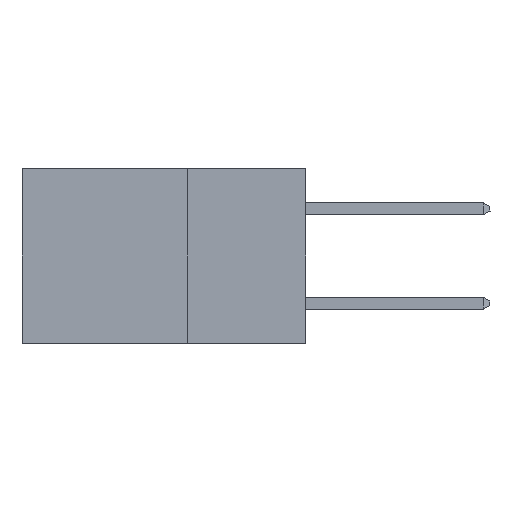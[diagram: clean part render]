
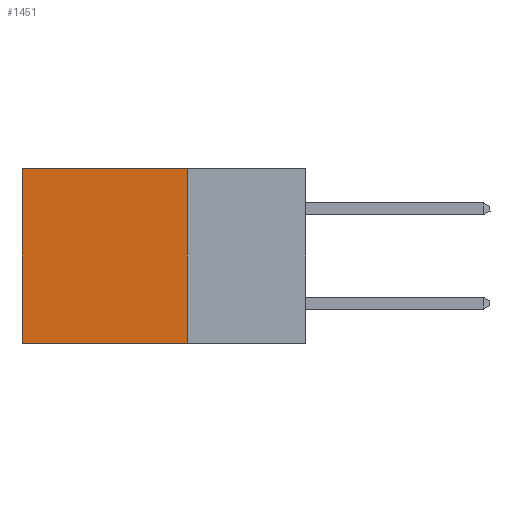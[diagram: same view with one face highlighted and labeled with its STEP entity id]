
A CAD part, left-side view. The second image highlights one B-rep face of the part: STEP entity #1451.
In plain terms, the highlighted planar face has unit normal (-1, 0, 0).
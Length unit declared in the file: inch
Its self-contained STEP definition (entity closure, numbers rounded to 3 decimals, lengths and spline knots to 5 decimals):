
#1451 = ADVANCED_FACE ( 'NONE', ( #2980 ), #4570, .F. ) ;
#2980 = FACE_OUTER_BOUND ( 'NONE', #17753, .T. ) ;
#3578 = VECTOR ( 'NONE', #20373, 39.37008 ) ;
#4069 = VERTEX_POINT ( 'NONE', #14468 ) ;
#4570 = PLANE ( 'NONE',  #22910 ) ;
#4605 = CARTESIAN_POINT ( 'NONE',  ( 0.298, 0.25, 0. ) ) ;
#6510 = VECTOR ( 'NONE', #19033, 39.37008 ) ;
#6691 = CARTESIAN_POINT ( 'NONE',  ( 0.298, 0.25, 0. ) ) ;
#6732 = DIRECTION ( 'NONE',  ( 0., 0., -1. ) ) ;
#6800 = DIRECTION ( 'NONE',  ( 1., 0., 0. ) ) ;
#7821 = EDGE_CURVE ( 'NONE', #13176, #16504, #13491, .T. ) ;
#8894 = CARTESIAN_POINT ( 'NONE',  ( 0.298, 0.6, 0. ) ) ;
#9764 = ORIENTED_EDGE ( 'NONE', *, *, #7821, .T. ) ;
#9885 = CARTESIAN_POINT ( 'NONE',  ( 0.298, 0.6, 0. ) ) ;
#10359 = CARTESIAN_POINT ( 'NONE',  ( 0.298, 0.25, -0.37 ) ) ;
#10582 = ORIENTED_EDGE ( 'NONE', *, *, #23614, .T. ) ;
#10862 = DIRECTION ( 'NONE',  ( 0., 0., -1. ) ) ;
#11301 = CARTESIAN_POINT ( 'NONE',  ( 0.298, 0.25, 0. ) ) ;
#11393 = LINE ( 'NONE', #10359, #17206 ) ;
#13176 = VERTEX_POINT ( 'NONE', #11301 ) ;
#13491 = LINE ( 'NONE', #6691, #3578 ) ;
#13542 = EDGE_CURVE ( 'NONE', #15235, #4069, #11393, .T. ) ;
#14468 = CARTESIAN_POINT ( 'NONE',  ( 0.298, 0.6, -0.37 ) ) ;
#15235 = VERTEX_POINT ( 'NONE', #23023 ) ;
#15592 = VECTOR ( 'NONE', #10862, 39.37008 ) ;
#16297 = EDGE_CURVE ( 'NONE', #13176, #15235, #16318, .T. ) ;
#16318 = LINE ( 'NONE', #20911, #6510 ) ;
#16504 = VERTEX_POINT ( 'NONE', #9885 ) ;
#17056 = ORIENTED_EDGE ( 'NONE', *, *, #16297, .F. ) ;
#17206 = VECTOR ( 'NONE', #23944, 39.37008 ) ;
#17753 = EDGE_LOOP ( 'NONE', ( #10582, #18983, #17056, #9764 ) ) ;
#18983 = ORIENTED_EDGE ( 'NONE', *, *, #13542, .F. ) ;
#19033 = DIRECTION ( 'NONE',  ( 0., 0., -1. ) ) ;
#20373 = DIRECTION ( 'NONE',  ( 0., 1., 0. ) ) ;
#20911 = CARTESIAN_POINT ( 'NONE',  ( 0.298, 0.25, 0. ) ) ;
#21977 = LINE ( 'NONE', #8894, #15592 ) ;
#22910 = AXIS2_PLACEMENT_3D ( 'NONE', #4605, #6800, #6732 ) ;
#23023 = CARTESIAN_POINT ( 'NONE',  ( 0.298, 0.25, -0.37 ) ) ;
#23614 = EDGE_CURVE ( 'NONE', #16504, #4069, #21977, .T. ) ;
#23944 = DIRECTION ( 'NONE',  ( 0., 1., 0. ) ) ;
